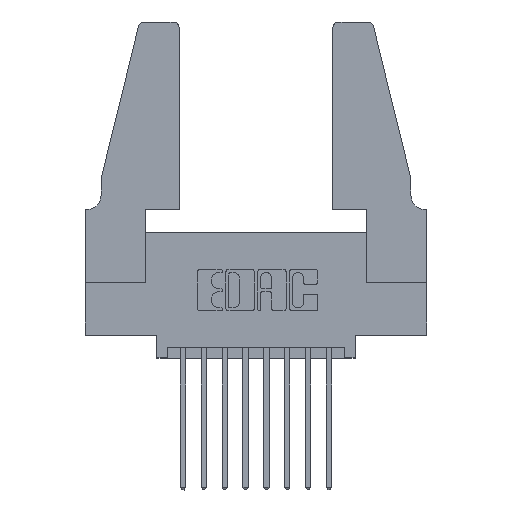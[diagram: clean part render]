
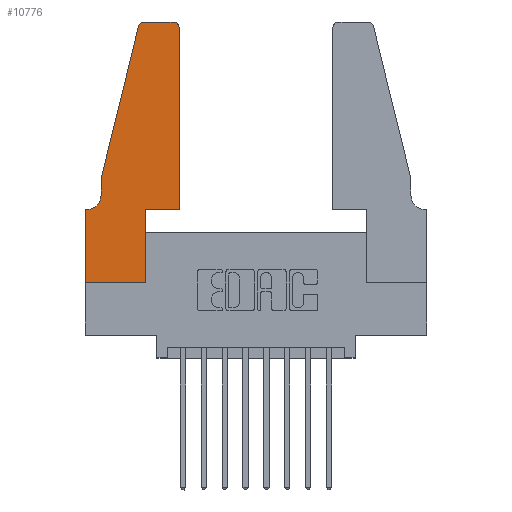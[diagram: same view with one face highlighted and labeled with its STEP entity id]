
A CAD part, top view. The second image highlights one B-rep face of the part: STEP entity #10776.
In plain terms, the highlighted planar face has unit normal (0, 0, 1).
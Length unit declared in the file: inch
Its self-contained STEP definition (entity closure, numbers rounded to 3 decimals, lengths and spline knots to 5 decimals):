
#12 = DIRECTION ( 'NONE',  ( 1., 0., 0. ) ) ;
#15 = ORIENTED_EDGE ( 'NONE', *, *, #7105, .T. ) ;
#101 = ORIENTED_EDGE ( 'NONE', *, *, #1064, .T. ) ;
#201 = VECTOR ( 'NONE', #12, 39.37008 ) ;
#497 = ORIENTED_EDGE ( 'NONE', *, *, #11747, .T. ) ;
#551 = VECTOR ( 'NONE', #753, 39.37008 ) ;
#695 = DIRECTION ( 'NONE',  ( -1., 0., 0. ) ) ;
#753 = DIRECTION ( 'NONE',  ( 0., -1., 0. ) ) ;
#836 = VERTEX_POINT ( 'NONE', #3162 ) ;
#888 = VECTOR ( 'NONE', #13124, 39.37008 ) ;
#933 = CARTESIAN_POINT ( 'NONE',  ( 0.4205, 1.22, 0.37 ) ) ;
#1025 = EDGE_CURVE ( 'NONE', #11677, #9592, #9315, .T. ) ;
#1038 = LINE ( 'NONE', #11746, #6266 ) ;
#1062 = EDGE_CURVE ( 'NONE', #7798, #4997, #3128, .T. ) ;
#1064 = EDGE_CURVE ( 'NONE', #2899, #7375, #1038, .T. ) ;
#1391 = VERTEX_POINT ( 'NONE', #3575 ) ;
#1756 = DIRECTION ( 'NONE',  ( -1., 0., 0. ) ) ;
#1901 = DIRECTION ( 'NONE',  ( 0., 0., 1. ) ) ;
#2003 = CARTESIAN_POINT ( 'NONE',  ( 0.0755, 0.35, 0.37 ) ) ;
#2118 = CARTESIAN_POINT ( 'NONE',  ( 0.4505, 0.35, 0.37 ) ) ;
#2441 = ORIENTED_EDGE ( 'NONE', *, *, #9099, .T. ) ;
#2544 = VECTOR ( 'NONE', #5452, 39.37008 ) ;
#2557 = ORIENTED_EDGE ( 'NONE', *, *, #8828, .T. ) ;
#2805 = AXIS2_PLACEMENT_3D ( 'NONE', #933, #1901, #10058 ) ;
#2899 = VERTEX_POINT ( 'NONE', #11942 ) ;
#2940 = CIRCLE ( 'NONE', #10620, 0.07 ) ;
#3122 = VECTOR ( 'NONE', #3515, 39.37008 ) ;
#3128 = LINE ( 'NONE', #11791, #4222 ) ;
#3162 = CARTESIAN_POINT ( 'NONE',  ( 0.2865, 0.35, 0.37 ) ) ;
#3253 = ORIENTED_EDGE ( 'NONE', *, *, #1025, .T. ) ;
#3326 = CARTESIAN_POINT ( 'NONE',  ( 0.4505, 0.35, 0.37 ) ) ;
#3407 = ORIENTED_EDGE ( 'NONE', *, *, #1062, .T. ) ;
#3515 = DIRECTION ( 'NONE',  ( 0., -1., 0. ) ) ;
#3564 = LINE ( 'NONE', #7909, #551 ) ;
#3575 = CARTESIAN_POINT ( 'NONE',  ( 0.0055, 0.35, 0.37 ) ) ;
#3644 = CARTESIAN_POINT ( 'NONE',  ( 0., 0., 0.37 ) ) ;
#3665 = ORIENTED_EDGE ( 'NONE', *, *, #10275, .T. ) ;
#3916 = CIRCLE ( 'NONE', #10185, 0.03 ) ;
#3959 = ORIENTED_EDGE ( 'NONE', *, *, #9942, .T. ) ;
#4207 = CARTESIAN_POINT ( 'NONE',  ( 0.2865, 0.35, 0.37 ) ) ;
#4222 = VECTOR ( 'NONE', #7754, 39.37008 ) ;
#4921 = CARTESIAN_POINT ( 'NONE',  ( 0.0755, 0.5, 0.37 ) ) ;
#4997 = VERTEX_POINT ( 'NONE', #4921 ) ;
#5128 = VERTEX_POINT ( 'NONE', #9718 ) ;
#5411 = LINE ( 'NONE', #8431, #2544 ) ;
#5452 = DIRECTION ( 'NONE',  ( 1., 0., 0. ) ) ;
#6200 = CARTESIAN_POINT ( 'NONE',  ( 0.4505, 1.22, 0.37 ) ) ;
#6266 = VECTOR ( 'NONE', #695, 39.37008 ) ;
#6536 = ORIENTED_EDGE ( 'NONE', *, *, #13167, .T. ) ;
#6770 = DIRECTION ( 'NONE',  ( 0., 1., 0. ) ) ;
#6935 = VERTEX_POINT ( 'NONE', #11055 ) ;
#7105 = EDGE_CURVE ( 'NONE', #5128, #836, #10973, .T. ) ;
#7349 = FACE_OUTER_BOUND ( 'NONE', #10692, .T. ) ;
#7375 = VERTEX_POINT ( 'NONE', #11907 ) ;
#7437 = DIRECTION ( 'NONE',  ( 0., 1., 0. ) ) ;
#7470 = CARTESIAN_POINT ( 'NONE',  ( 0.25487, 1.22718, 0.37 ) ) ;
#7754 = DIRECTION ( 'NONE',  ( -0.239, -0.971, 0. ) ) ;
#7798 = VERTEX_POINT ( 'NONE', #7470 ) ;
#7864 = DIRECTION ( 'NONE',  ( 0., 0., -1. ) ) ;
#7909 = CARTESIAN_POINT ( 'NONE',  ( 0.0755, 0.5, 0.37 ) ) ;
#7989 = VERTEX_POINT ( 'NONE', #3644 ) ;
#8108 = CIRCLE ( 'NONE', #2805, 0.03 ) ;
#8134 = ORIENTED_EDGE ( 'NONE', *, *, #8675, .T. ) ;
#8157 = DIRECTION ( 'NONE',  ( 1., 0., 0. ) ) ;
#8188 = ORIENTED_EDGE ( 'NONE', *, *, #9941, .T. ) ;
#8431 = CARTESIAN_POINT ( 'NONE',  ( 0., 0., 0.37 ) ) ;
#8675 = EDGE_CURVE ( 'NONE', #7375, #7798, #3916, .T. ) ;
#8828 = EDGE_CURVE ( 'NONE', #1391, #10722, #10611, .T. ) ;
#8972 = CARTESIAN_POINT ( 'NONE',  ( 0.284, 1.22, 0.37 ) ) ;
#9099 = EDGE_CURVE ( 'NONE', #10722, #7989, #11412, .T. ) ;
#9191 = VECTOR ( 'NONE', #7437, 39.37008 ) ;
#9315 = LINE ( 'NONE', #12866, #12963 ) ;
#9338 = AXIS2_PLACEMENT_3D ( 'NONE', #13122, #13156, #8157 ) ;
#9592 = VERTEX_POINT ( 'NONE', #6200 ) ;
#9718 = CARTESIAN_POINT ( 'NONE',  ( 0.2865, 0., 0.37 ) ) ;
#9941 = EDGE_CURVE ( 'NONE', #6935, #1391, #2940, .T. ) ;
#9942 = EDGE_CURVE ( 'NONE', #4997, #6935, #3564, .T. ) ;
#10058 = DIRECTION ( 'NONE',  ( 1., 0., 0. ) ) ;
#10071 = PLANE ( 'NONE',  #9338 ) ;
#10185 = AXIS2_PLACEMENT_3D ( 'NONE', #8972, #11043, #11738 ) ;
#10275 = EDGE_CURVE ( 'NONE', #836, #11677, #13089, .T. ) ;
#10611 = LINE ( 'NONE', #2003, #888 ) ;
#10620 = AXIS2_PLACEMENT_3D ( 'NONE', #12923, #7864, #1756 ) ;
#10692 = EDGE_LOOP ( 'NONE', ( #101, #8134, #3407, #3959, #8188, #2557, #2441, #497, #15, #3665, #3253, #6536 ) ) ;
#10722 = VERTEX_POINT ( 'NONE', #13037 ) ;
#10776 = ADVANCED_FACE ( 'NONE', ( #7349 ), #10071, .T. ) ;
#10973 = LINE ( 'NONE', #4207, #9191 ) ;
#11043 = DIRECTION ( 'NONE',  ( 0., 0., 1. ) ) ;
#11055 = CARTESIAN_POINT ( 'NONE',  ( 0.0755, 0.42, 0.37 ) ) ;
#11412 = LINE ( 'NONE', #12547, #3122 ) ;
#11677 = VERTEX_POINT ( 'NONE', #3326 ) ;
#11738 = DIRECTION ( 'NONE',  ( 1., 0., 0. ) ) ;
#11746 = CARTESIAN_POINT ( 'NONE',  ( 0.2605, 1.25, 0.37 ) ) ;
#11747 = EDGE_CURVE ( 'NONE', #7989, #5128, #5411, .T. ) ;
#11791 = CARTESIAN_POINT ( 'NONE',  ( 0.0755, 0.5, 0.37 ) ) ;
#11907 = CARTESIAN_POINT ( 'NONE',  ( 0.284, 1.25, 0.37 ) ) ;
#11942 = CARTESIAN_POINT ( 'NONE',  ( 0.4205, 1.25, 0.37 ) ) ;
#12547 = CARTESIAN_POINT ( 'NONE',  ( 0., 0., 0.37 ) ) ;
#12866 = CARTESIAN_POINT ( 'NONE',  ( 0.4505, 0.35, 0.37 ) ) ;
#12923 = CARTESIAN_POINT ( 'NONE',  ( 0.0055, 0.42, 0.37 ) ) ;
#12963 = VECTOR ( 'NONE', #6770, 39.37008 ) ;
#13037 = CARTESIAN_POINT ( 'NONE',  ( 0., 0.35, 0.37 ) ) ;
#13089 = LINE ( 'NONE', #2118, #201 ) ;
#13122 = CARTESIAN_POINT ( 'NONE',  ( 0., 0.35, 0.37 ) ) ;
#13124 = DIRECTION ( 'NONE',  ( -1., 0., 0. ) ) ;
#13156 = DIRECTION ( 'NONE',  ( 0., 0., 1. ) ) ;
#13167 = EDGE_CURVE ( 'NONE', #9592, #2899, #8108, .T. ) ;
